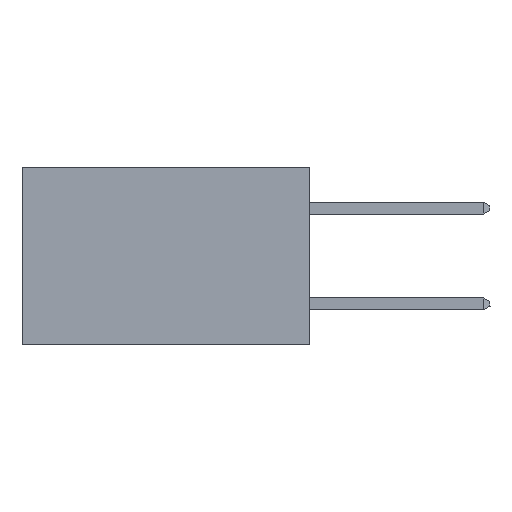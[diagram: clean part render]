
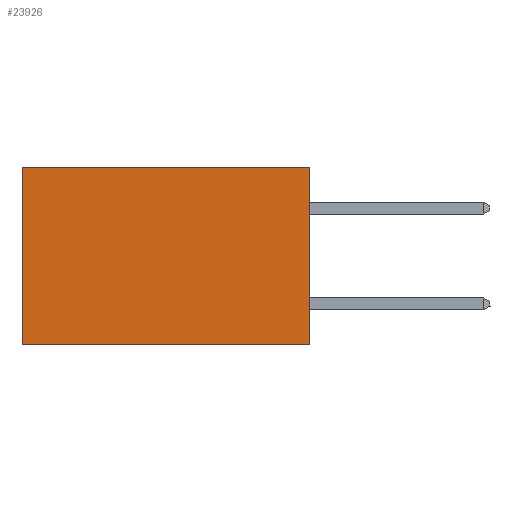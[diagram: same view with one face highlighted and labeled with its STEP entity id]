
A CAD part, left-side view. The second image highlights one B-rep face of the part: STEP entity #23926.
In plain terms, the highlighted planar face has unit normal (-1, 0, 0).
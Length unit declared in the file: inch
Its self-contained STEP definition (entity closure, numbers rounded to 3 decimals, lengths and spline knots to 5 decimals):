
#195 = VECTOR ( 'NONE', #21260, 39.37008 ) ;
#299 = CARTESIAN_POINT ( 'NONE',  ( 0.2875, 0., 0. ) ) ;
#323 = LINE ( 'NONE', #32456, #41085 ) ;
#7727 = DIRECTION ( 'NONE',  ( 0., 0., -1. ) ) ;
#9603 = LINE ( 'NONE', #299, #15576 ) ;
#13911 = VECTOR ( 'NONE', #7727, 39.37008 ) ;
#14802 = CARTESIAN_POINT ( 'NONE',  ( 0.2875, 0.6, 0. ) ) ;
#15431 = ORIENTED_EDGE ( 'NONE', *, *, #25883, .F. ) ;
#15576 = VECTOR ( 'NONE', #22512, 39.37008 ) ;
#16947 = EDGE_LOOP ( 'NONE', ( #20203, #15431, #36215, #25151 ) ) ;
#17081 = VERTEX_POINT ( 'NONE', #30521 ) ;
#18039 = LINE ( 'NONE', #18045, #195 ) ;
#18045 = CARTESIAN_POINT ( 'NONE',  ( 0.2875, 0., 0. ) ) ;
#19935 = CARTESIAN_POINT ( 'NONE',  ( 0.2875, 0.6, 0. ) ) ;
#20203 = ORIENTED_EDGE ( 'NONE', *, *, #37067, .T. ) ;
#20565 = PLANE ( 'NONE',  #28538 ) ;
#20592 = CARTESIAN_POINT ( 'NONE',  ( 0.2875, 0., 0. ) ) ;
#21125 = DIRECTION ( 'NONE',  ( 0., 0., -1. ) ) ;
#21260 = DIRECTION ( 'NONE',  ( 0., 1., 0. ) ) ;
#22125 = EDGE_CURVE ( 'NONE', #32164, #35285, #18039, .T. ) ;
#22377 = EDGE_CURVE ( 'NONE', #32164, #17081, #9603, .T. ) ;
#22512 = DIRECTION ( 'NONE',  ( 0., 0., -1. ) ) ;
#23926 = ADVANCED_FACE ( 'NONE', ( #26839 ), #20565, .F. ) ;
#25151 = ORIENTED_EDGE ( 'NONE', *, *, #22125, .T. ) ;
#25849 = VERTEX_POINT ( 'NONE', #32305 ) ;
#25883 = EDGE_CURVE ( 'NONE', #17081, #25849, #323, .T. ) ;
#26839 = FACE_OUTER_BOUND ( 'NONE', #16947, .T. ) ;
#28538 = AXIS2_PLACEMENT_3D ( 'NONE', #30597, #37065, #21125 ) ;
#30521 = CARTESIAN_POINT ( 'NONE',  ( 0.2875, 0., -0.37 ) ) ;
#30597 = CARTESIAN_POINT ( 'NONE',  ( 0.2875, 0., 0. ) ) ;
#32164 = VERTEX_POINT ( 'NONE', #20592 ) ;
#32305 = CARTESIAN_POINT ( 'NONE',  ( 0.2875, 0.6, -0.37 ) ) ;
#32456 = CARTESIAN_POINT ( 'NONE',  ( 0.2875, 0., -0.37 ) ) ;
#34856 = LINE ( 'NONE', #19935, #13911 ) ;
#35285 = VERTEX_POINT ( 'NONE', #14802 ) ;
#36215 = ORIENTED_EDGE ( 'NONE', *, *, #22377, .F. ) ;
#37065 = DIRECTION ( 'NONE',  ( 1., 0., 0. ) ) ;
#37067 = EDGE_CURVE ( 'NONE', #35285, #25849, #34856, .T. ) ;
#39032 = DIRECTION ( 'NONE',  ( 0., 1., 0. ) ) ;
#41085 = VECTOR ( 'NONE', #39032, 39.37008 ) ;
